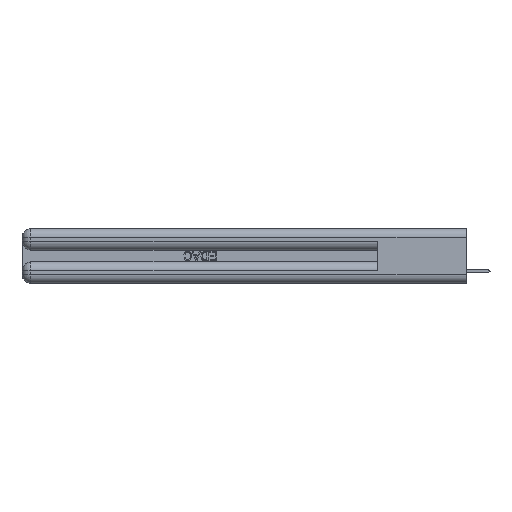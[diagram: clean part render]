
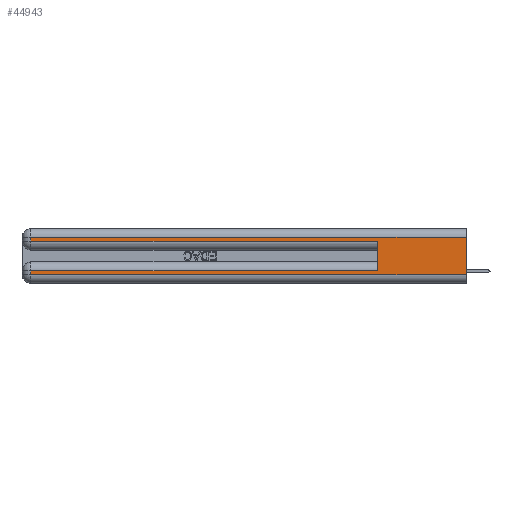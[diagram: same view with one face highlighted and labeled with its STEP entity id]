
A CAD part, left-side view. The second image highlights one B-rep face of the part: STEP entity #44943.
In plain terms, the highlighted planar face has unit normal (-1, 0, 0).
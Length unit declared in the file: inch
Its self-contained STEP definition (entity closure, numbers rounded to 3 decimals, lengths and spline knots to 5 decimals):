
#31 = EDGE_CURVE ( 'NONE', #39283, #38810, #30591, .T. ) ;
#262 = EDGE_CURVE ( 'NONE', #45140, #26480, #5447, .T. ) ;
#846 = CARTESIAN_POINT ( 'NONE',  ( 0., 2.94, 0.37 ) ) ;
#996 = CARTESIAN_POINT ( 'NONE',  ( 0., 0.6, 0.285 ) ) ;
#1023 = ORIENTED_EDGE ( 'NONE', *, *, #26195, .F. ) ;
#1666 = ORIENTED_EDGE ( 'NONE', *, *, #43226, .T. ) ;
#1907 = DIRECTION ( 'NONE',  ( 0., -1., 0. ) ) ;
#1964 = LINE ( 'NONE', #7755, #11945 ) ;
#2141 = EDGE_CURVE ( 'NONE', #38810, #22865, #40716, .T. ) ;
#2150 = VECTOR ( 'NONE', #14911, 39.37008 ) ;
#3808 = LINE ( 'NONE', #32944, #10576 ) ;
#4833 = FACE_OUTER_BOUND ( 'NONE', #45696, .T. ) ;
#5052 = ORIENTED_EDGE ( 'NONE', *, *, #29686, .F. ) ;
#5447 = LINE ( 'NONE', #16138, #30554 ) ;
#6433 = CARTESIAN_POINT ( 'NONE',  ( 0., 0., 0.31 ) ) ;
#7755 = CARTESIAN_POINT ( 'NONE',  ( 0., 0.6, 0.145 ) ) ;
#8209 = ORIENTED_EDGE ( 'NONE', *, *, #31, .T. ) ;
#9090 = LINE ( 'NONE', #26713, #35315 ) ;
#10576 = VECTOR ( 'NONE', #22543, 39.37008 ) ;
#11945 = VECTOR ( 'NONE', #25423, 39.37008 ) ;
#13741 = ORIENTED_EDGE ( 'NONE', *, *, #18523, .T. ) ;
#14146 = CARTESIAN_POINT ( 'NONE',  ( 0., 2.94, 0.31 ) ) ;
#14223 = ORIENTED_EDGE ( 'NONE', *, *, #33653, .T. ) ;
#14605 = CARTESIAN_POINT ( 'NONE',  ( 0., 0., 0.31 ) ) ;
#14911 = DIRECTION ( 'NONE',  ( 0., 1., 0. ) ) ;
#15010 = CARTESIAN_POINT ( 'NONE',  ( 0., 0., 0.085 ) ) ;
#15196 = VECTOR ( 'NONE', #25822, 39.37008 ) ;
#16026 = CARTESIAN_POINT ( 'NONE',  ( 0., 2.94, 0.06 ) ) ;
#16138 = CARTESIAN_POINT ( 'NONE',  ( 0., 2.94, 0.37 ) ) ;
#18405 = CARTESIAN_POINT ( 'NONE',  ( 0., 0., 0.37 ) ) ;
#18523 = EDGE_CURVE ( 'NONE', #43287, #45140, #26482, .T. ) ;
#19534 = CARTESIAN_POINT ( 'NONE',  ( 0., 2.94, 0.285 ) ) ;
#22031 = PLANE ( 'NONE',  #40686 ) ;
#22543 = DIRECTION ( 'NONE',  ( 0., 0., -1. ) ) ;
#22865 = VERTEX_POINT ( 'NONE', #19534 ) ;
#22994 = VERTEX_POINT ( 'NONE', #996 ) ;
#24683 = ORIENTED_EDGE ( 'NONE', *, *, #2141, .T. ) ;
#24710 = VERTEX_POINT ( 'NONE', #33606 ) ;
#25423 = DIRECTION ( 'NONE',  ( 0., 0., 1. ) ) ;
#25822 = DIRECTION ( 'NONE',  ( 0., 0., -1. ) ) ;
#26195 = EDGE_CURVE ( 'NONE', #43287, #22994, #1964, .T. ) ;
#26375 = CARTESIAN_POINT ( 'NONE',  ( 0., 2.94, 0.085 ) ) ;
#26480 = VERTEX_POINT ( 'NONE', #16026 ) ;
#26482 = LINE ( 'NONE', #15010, #34817 ) ;
#26713 = CARTESIAN_POINT ( 'NONE',  ( 0., 0., 0.06 ) ) ;
#26903 = DIRECTION ( 'NONE',  ( 0., 0., -1. ) ) ;
#28864 = LINE ( 'NONE', #41077, #41004 ) ;
#29686 = EDGE_CURVE ( 'NONE', #39283, #24710, #3808, .T. ) ;
#30554 = VECTOR ( 'NONE', #26903, 39.37008 ) ;
#30591 = LINE ( 'NONE', #14605, #2150 ) ;
#31043 = DIRECTION ( 'NONE',  ( 0., -1., 0. ) ) ;
#32944 = CARTESIAN_POINT ( 'NONE',  ( 0., 0., 0.37 ) ) ;
#33606 = CARTESIAN_POINT ( 'NONE',  ( 0., 0., 0.06 ) ) ;
#33653 = EDGE_CURVE ( 'NONE', #22865, #22994, #28864, .T. ) ;
#34817 = VECTOR ( 'NONE', #39848, 39.37008 ) ;
#35115 = ORIENTED_EDGE ( 'NONE', *, *, #262, .T. ) ;
#35315 = VECTOR ( 'NONE', #1907, 39.37008 ) ;
#35848 = DIRECTION ( 'NONE',  ( 1., 0., 0. ) ) ;
#38810 = VERTEX_POINT ( 'NONE', #14146 ) ;
#39283 = VERTEX_POINT ( 'NONE', #6433 ) ;
#39370 = DIRECTION ( 'NONE',  ( 0., 0., -1. ) ) ;
#39848 = DIRECTION ( 'NONE',  ( 0., 1., 0. ) ) ;
#40686 = AXIS2_PLACEMENT_3D ( 'NONE', #18405, #35848, #39370 ) ;
#40716 = LINE ( 'NONE', #846, #15196 ) ;
#41004 = VECTOR ( 'NONE', #31043, 39.37008 ) ;
#41077 = CARTESIAN_POINT ( 'NONE',  ( 0., 0., 0.285 ) ) ;
#41872 = CARTESIAN_POINT ( 'NONE',  ( 0., 0.6, 0.085 ) ) ;
#43226 = EDGE_CURVE ( 'NONE', #26480, #24710, #9090, .T. ) ;
#43287 = VERTEX_POINT ( 'NONE', #41872 ) ;
#44943 = ADVANCED_FACE ( 'NONE', ( #4833 ), #22031, .F. ) ;
#45140 = VERTEX_POINT ( 'NONE', #26375 ) ;
#45696 = EDGE_LOOP ( 'NONE', ( #5052, #8209, #24683, #14223, #1023, #13741, #35115, #1666 ) ) ;
